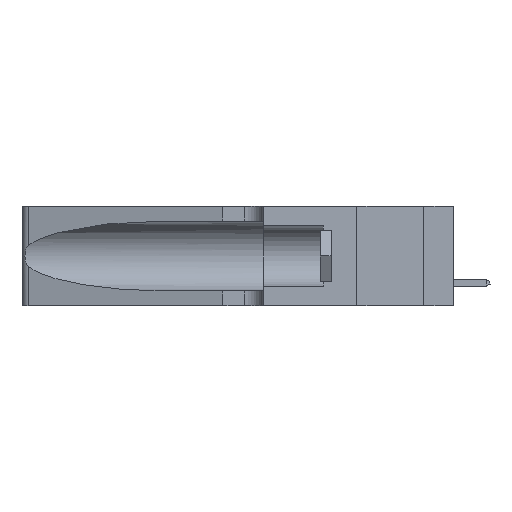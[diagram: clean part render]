
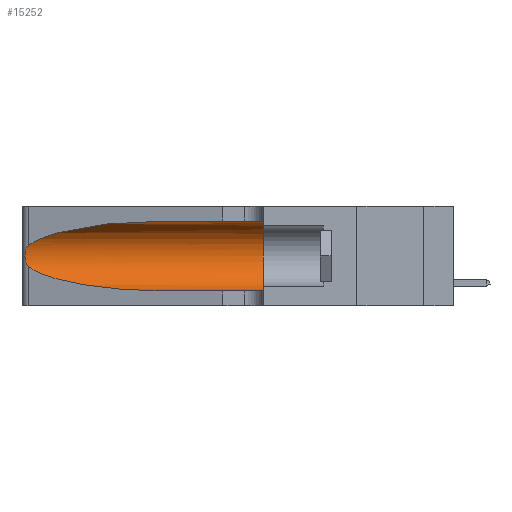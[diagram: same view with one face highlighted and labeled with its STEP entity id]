
A CAD part, left-side view. The second image highlights one B-rep face of the part: STEP entity #15252.
In plain terms, the highlighted cylindrical face has radius 3.308 mm (diameter 6.617 mm), a partial arc.
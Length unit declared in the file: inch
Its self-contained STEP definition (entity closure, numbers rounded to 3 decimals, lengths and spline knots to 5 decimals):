
#680 = CARTESIAN_POINT ( 'NONE',  ( 0.18966, 0.96281, 0.31525 ) ) ;
#1434 = FACE_OUTER_BOUND ( 'NONE', #25936, .T. ) ;
#3423 = CARTESIAN_POINT ( 'NONE',  ( 0.25639, 1.23184, 0.21858 ) ) ;
#3550 = CARTESIAN_POINT ( 'NONE',  ( 0.2373, 1.15595, 0.08982 ) ) ;
#3742 = VECTOR ( 'NONE', #4199, 39.37008 ) ;
#4199 = DIRECTION ( 'NONE',  ( 0., -1., 0. ) ) ;
#4414 = VERTEX_POINT ( 'NONE', #16970 ) ;
#4445 = CARTESIAN_POINT ( 'NONE',  ( 0.1305, 0.72297, 0.05475 ) ) ;
#4825 = CARTESIAN_POINT ( 'NONE',  ( 0.1305, 0.72297, 0.31525 ) ) ;
#4848 = DIRECTION ( 'NONE',  ( 0., 1., 0. ) ) ;
#4968 = DIRECTION ( 'NONE',  ( 0., 0., -1. ) ) ;
#5951 = CARTESIAN_POINT ( 'NONE',  ( 0.26018, 1.23835, 0.19895 ) ) ;
#6071 = EDGE_CURVE ( 'NONE', #14697, #8524, #29322, .T. ) ;
#6518 = EDGE_CURVE ( 'NONE', #34150, #15717, #10079, .T. ) ;
#6553 = DIRECTION ( 'NONE',  ( 0., -1., 0. ) ) ;
#6940 = CARTESIAN_POINT ( 'NONE',  ( 0.2373, 1.15595, 0.28018 ) ) ;
#7814 = ORIENTED_EDGE ( 'NONE', *, *, #6518, .T. ) ;
#7824 = ORIENTED_EDGE ( 'NONE', *, *, #25787, .F. ) ;
#8524 = VERTEX_POINT ( 'NONE', #13224 ) ;
#8774 = CARTESIAN_POINT ( 'NONE',  ( 0.25639, 1.23186, 0.15144 ) ) ;
#10079 = B_SPLINE_CURVE_WITH_KNOTS ( 'NONE', 3,
 ( #28839, #22294, #3423, #18648, #21967, #5951, #31752, #43363, #19350, #23769, #20417, #8774, #36712, #43868 ),
 .UNSPECIFIED., .F., .F.,
 ( 4, 2, 2, 2, 2, 2, 4 ),
 ( 0., 0.00027, 0.00053, 0.00107, 0.0016, 0.00187, 0.00214 ),
 .UNSPECIFIED. ) ;
#10086 = CARTESIAN_POINT ( 'NONE',  ( 0.25487, 1.22718, 0.14631 ) ) ;
#11390 = CARTESIAN_POINT ( 'NONE',  ( 0.1305, 1.61858, 0.185 ) ) ;
#12326 = ORIENTED_EDGE ( 'NONE', *, *, #6071, .F. ) ;
#12919 = CYLINDRICAL_SURFACE ( 'NONE', #24112, 0.13025 ) ;
#13224 = CARTESIAN_POINT ( 'NONE',  ( 0.1305, 0.35, 0.31525 ) ) ;
#14605 = CARTESIAN_POINT ( 'NONE',  ( 0.25487, 1.22718, 0.22369 ) ) ;
#14697 = VERTEX_POINT ( 'NONE', #4825 ) ;
#15252 = ADVANCED_FACE ( 'NONE', ( #1434 ), #12919, .F. ) ;
#15717 = VERTEX_POINT ( 'NONE', #10086 ) ;
#16970 = CARTESIAN_POINT ( 'NONE',  ( 0.1305, 0.35, 0.05475 ) ) ;
#17080 = CARTESIAN_POINT ( 'NONE',  ( 0.25487, 1.22718, 0.22369 ) ) ;
#17918 = VERTEX_POINT ( 'NONE', #25630 ) ;
#18116 = EDGE_CURVE ( 'NONE', #14697, #34150, #39025, .T. ) ;
#18648 = CARTESIAN_POINT ( 'NONE',  ( 0.25787, 1.23484, 0.2124 ) ) ;
#19350 = CARTESIAN_POINT ( 'NONE',  ( 0.26017, 1.23833, 0.17102 ) ) ;
#20417 = CARTESIAN_POINT ( 'NONE',  ( 0.25789, 1.23486, 0.15765 ) ) ;
#20701 = CARTESIAN_POINT ( 'NONE',  ( 0.1305, 1.61858, 0.05475 ) ) ;
#21967 = CARTESIAN_POINT ( 'NONE',  ( 0.25854, 1.2359, 0.20912 ) ) ;
#22267 = VECTOR ( 'NONE', #6553, 39.37008 ) ;
#22294 = CARTESIAN_POINT ( 'NONE',  ( 0.25555, 1.22994, 0.2215 ) ) ;
#22995 = EDGE_CURVE ( 'NONE', #17918, #4414, #26655, .T. ) ;
#23769 = CARTESIAN_POINT ( 'NONE',  ( 0.25856, 1.23593, 0.16098 ) ) ;
#24112 = AXIS2_PLACEMENT_3D ( 'NONE', #11390, #39187, #4968 ) ;
#24384 = CARTESIAN_POINT ( 'NONE',  ( 0.25487, 1.22718, 0.14631 ) ) ;
#24567 = CARTESIAN_POINT ( 'NONE',  ( 0.1305, 1.61858, 0.31525 ) ) ;
#25630 = CARTESIAN_POINT ( 'NONE',  ( 0.1305, 0.72297, 0.05475 ) ) ;
#25787 = EDGE_CURVE ( 'NONE', #8524, #4414, #32988, .T. ) ;
#25882 = AXIS2_PLACEMENT_3D ( 'NONE', #38304, #4848, #29338 ) ;
#25936 = EDGE_LOOP ( 'NONE', ( #43045, #7814, #30180, #26150, #7824, #12326 ) ) ;
#26150 = ORIENTED_EDGE ( 'NONE', *, *, #22995, .T. ) ;
#26655 = LINE ( 'NONE', #20701, #22267 ) ;
#28839 = CARTESIAN_POINT ( 'NONE',  ( 0.25487, 1.22718, 0.22369 ) ) ;
#29150 = CARTESIAN_POINT ( 'NONE',  ( 0.1305, 0.72297, 0.31525 ) ) ;
#29322 = LINE ( 'NONE', #24567, #3742 ) ;
#29338 = DIRECTION ( 'NONE',  ( 0., 0., 1. ) ) ;
#29576 =( BOUNDED_CURVE ( )  B_SPLINE_CURVE ( 3, ( #24384, #3550, #43214, #4445 ),
 .UNSPECIFIED., .F., .F. ) 
 B_SPLINE_CURVE_WITH_KNOTS ( ( 4, 4 ),
 ( 3.44316, 4.71239 ),
 .UNSPECIFIED. ) 
 CURVE ( )  GEOMETRIC_REPRESENTATION_ITEM ( )  RATIONAL_B_SPLINE_CURVE ( ( 1., 0.87, 0.87, 1. ) ) 
 REPRESENTATION_ITEM ( '' )  );
#30180 = ORIENTED_EDGE ( 'NONE', *, *, #39792, .T. ) ;
#31752 = CARTESIAN_POINT ( 'NONE',  ( 0.26075, 1.23896, 0.19203 ) ) ;
#32988 = CIRCLE ( 'NONE', #25882, 0.13025 ) ;
#34150 = VERTEX_POINT ( 'NONE', #14605 ) ;
#36712 = CARTESIAN_POINT ( 'NONE',  ( 0.25555, 1.22993, 0.14849 ) ) ;
#38304 = CARTESIAN_POINT ( 'NONE',  ( 0.1305, 0.35, 0.185 ) ) ;
#39025 =( BOUNDED_CURVE ( )  B_SPLINE_CURVE ( 3, ( #29150, #680, #6940, #17080 ),
 .UNSPECIFIED., .F., .T. ) 
 B_SPLINE_CURVE_WITH_KNOTS ( ( 4, 4 ),
 ( 1.5708, 2.84003 ),
 .UNSPECIFIED. ) 
 CURVE ( )  GEOMETRIC_REPRESENTATION_ITEM ( )  RATIONAL_B_SPLINE_CURVE ( ( 1., 0.87, 0.87, 1. ) ) 
 REPRESENTATION_ITEM ( '' )  );
#39187 = DIRECTION ( 'NONE',  ( 0., -1., 0. ) ) ;
#39792 = EDGE_CURVE ( 'NONE', #15717, #17918, #29576, .T. ) ;
#43045 = ORIENTED_EDGE ( 'NONE', *, *, #18116, .T. ) ;
#43214 = CARTESIAN_POINT ( 'NONE',  ( 0.18966, 0.96281, 0.05475 ) ) ;
#43363 = CARTESIAN_POINT ( 'NONE',  ( 0.26075, 1.23896, 0.178 ) ) ;
#43868 = CARTESIAN_POINT ( 'NONE',  ( 0.25487, 1.22718, 0.14631 ) ) ;
